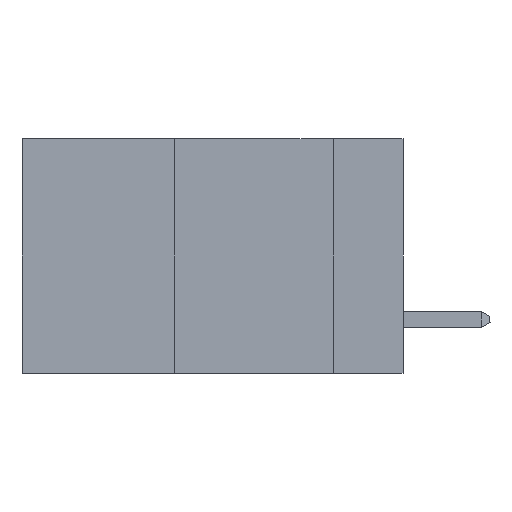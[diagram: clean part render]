
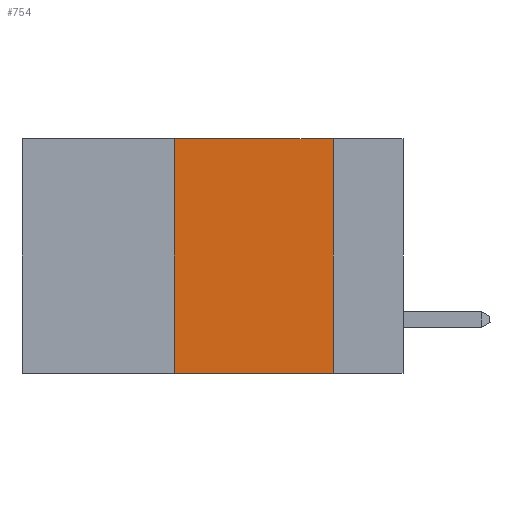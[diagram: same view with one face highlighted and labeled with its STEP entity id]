
A CAD part, left-side view. The second image highlights one B-rep face of the part: STEP entity #754.
In plain terms, the highlighted planar face has unit normal (-1, 0, 0).
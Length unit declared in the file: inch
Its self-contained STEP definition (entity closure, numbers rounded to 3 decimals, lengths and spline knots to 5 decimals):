
#645 = VECTOR ( 'NONE', #36175, 39.37008 ) ;
#754 = ADVANCED_FACE ( 'NONE', ( #48978 ), #19077, .F. ) ;
#2456 = CARTESIAN_POINT ( 'NONE',  ( 0., 0.11, 0. ) ) ;
#2941 = CARTESIAN_POINT ( 'NONE',  ( 0., 0.36, -0.37 ) ) ;
#5980 = CARTESIAN_POINT ( 'NONE',  ( 0., 0.11, -0.37 ) ) ;
#7815 = CARTESIAN_POINT ( 'NONE',  ( 0., 0.6, 0. ) ) ;
#9165 = CARTESIAN_POINT ( 'NONE',  ( 0., 0.6, 0. ) ) ;
#13330 = DIRECTION ( 'NONE',  ( 0., -1., 0. ) ) ;
#14213 = DIRECTION ( 'NONE',  ( 0., 0., -1. ) ) ;
#14962 = DIRECTION ( 'NONE',  ( 0., 0., 1. ) ) ;
#17615 = EDGE_CURVE ( 'NONE', #28993, #41306, #38905, .T. ) ;
#18755 = EDGE_CURVE ( 'NONE', #46736, #41306, #45353, .T. ) ;
#18777 = VECTOR ( 'NONE', #14213, 39.37008 ) ;
#19077 = PLANE ( 'NONE',  #19554 ) ;
#19101 = VERTEX_POINT ( 'NONE', #40124 ) ;
#19554 = AXIS2_PLACEMENT_3D ( 'NONE', #7815, #30616, #34260 ) ;
#22529 = ORIENTED_EDGE ( 'NONE', *, *, #38895, .F. ) ;
#28521 = EDGE_LOOP ( 'NONE', ( #42370, #34855, #22529, #30808 ) ) ;
#28993 = VERTEX_POINT ( 'NONE', #2456 ) ;
#29603 = VECTOR ( 'NONE', #14962, 39.37008 ) ;
#30616 = DIRECTION ( 'NONE',  ( 1., 0., 0. ) ) ;
#30808 = ORIENTED_EDGE ( 'NONE', *, *, #18755, .T. ) ;
#30868 = LINE ( 'NONE', #9165, #645 ) ;
#33307 = EDGE_CURVE ( 'NONE', #19101, #28993, #30868, .T. ) ;
#33642 = CARTESIAN_POINT ( 'NONE',  ( 0., 0.36, 0. ) ) ;
#34260 = DIRECTION ( 'NONE',  ( 0., 0., -1. ) ) ;
#34855 = ORIENTED_EDGE ( 'NONE', *, *, #33307, .F. ) ;
#35464 = LINE ( 'NONE', #33642, #29603 ) ;
#36175 = DIRECTION ( 'NONE',  ( 0., -1., 0. ) ) ;
#36565 = CARTESIAN_POINT ( 'NONE',  ( 0., 0.11, 0. ) ) ;
#37434 = CARTESIAN_POINT ( 'NONE',  ( 0., 0.6, -0.37 ) ) ;
#38895 = EDGE_CURVE ( 'NONE', #46736, #19101, #35464, .T. ) ;
#38905 = LINE ( 'NONE', #36565, #18777 ) ;
#40124 = CARTESIAN_POINT ( 'NONE',  ( 0., 0.36, 0. ) ) ;
#41271 = VECTOR ( 'NONE', #13330, 39.37008 ) ;
#41306 = VERTEX_POINT ( 'NONE', #5980 ) ;
#42370 = ORIENTED_EDGE ( 'NONE', *, *, #17615, .F. ) ;
#45353 = LINE ( 'NONE', #37434, #41271 ) ;
#46736 = VERTEX_POINT ( 'NONE', #2941 ) ;
#48978 = FACE_OUTER_BOUND ( 'NONE', #28521, .T. ) ;
